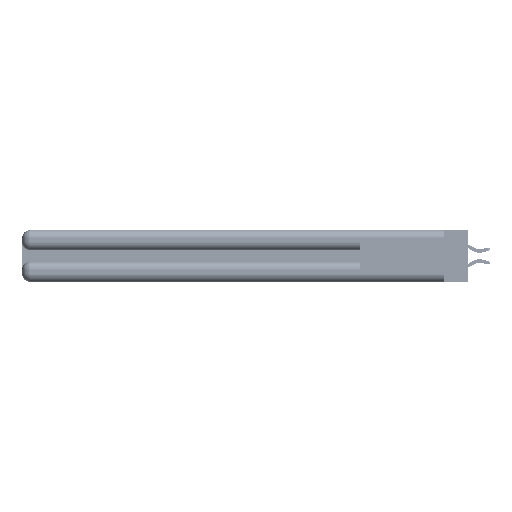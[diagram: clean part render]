
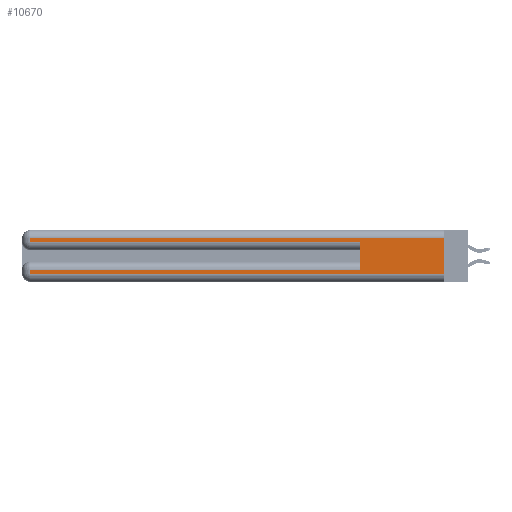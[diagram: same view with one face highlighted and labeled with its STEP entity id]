
A CAD part, left-side view. The second image highlights one B-rep face of the part: STEP entity #10670.
In plain terms, the highlighted planar face has unit normal (-1, 0, 0).
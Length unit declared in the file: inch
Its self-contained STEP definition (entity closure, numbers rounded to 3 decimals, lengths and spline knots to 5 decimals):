
#1679 = VECTOR ( 'NONE', #37091, 39.37008 ) ;
#2546 = VERTEX_POINT ( 'NONE', #47891 ) ;
#4419 = LINE ( 'NONE', #30171, #14768 ) ;
#5104 = ORIENTED_EDGE ( 'NONE', *, *, #55584, .T. ) ;
#5955 = LINE ( 'NONE', #19598, #27878 ) ;
#6009 = VERTEX_POINT ( 'NONE', #10461 ) ;
#6026 = LINE ( 'NONE', #41422, #39527 ) ;
#7440 = LINE ( 'NONE', #43760, #29347 ) ;
#9182 = EDGE_LOOP ( 'NONE', ( #13425, #17694, #44056, #31482, #10228, #5104, #28020, #56141 ) ) ;
#9237 = CARTESIAN_POINT ( 'NONE',  ( 0., 2.94, 0.06 ) ) ;
#10228 = ORIENTED_EDGE ( 'NONE', *, *, #19176, .F. ) ;
#10363 = VERTEX_POINT ( 'NONE', #9237 ) ;
#10461 = CARTESIAN_POINT ( 'NONE',  ( 0., 0.6, 0.285 ) ) ;
#10521 = VERTEX_POINT ( 'NONE', #23574 ) ;
#10670 = ADVANCED_FACE ( 'NONE', ( #22972 ), #11326, .F. ) ;
#11326 = PLANE ( 'NONE',  #25220 ) ;
#13425 = ORIENTED_EDGE ( 'NONE', *, *, #25751, .F. ) ;
#14768 = VECTOR ( 'NONE', #17001, 39.37008 ) ;
#15258 = VECTOR ( 'NONE', #37832, 39.37008 ) ;
#16600 = LINE ( 'NONE', #33447, #15258 ) ;
#16718 = VECTOR ( 'NONE', #22267, 39.37008 ) ;
#17001 = DIRECTION ( 'NONE',  ( 0., 1., 0. ) ) ;
#17694 = ORIENTED_EDGE ( 'NONE', *, *, #53744, .T. ) ;
#19176 = EDGE_CURVE ( 'NONE', #2546, #6009, #6026, .T. ) ;
#19598 = CARTESIAN_POINT ( 'NONE',  ( 0., 2.94, 0.37 ) ) ;
#20478 = VECTOR ( 'NONE', #41008, 39.37008 ) ;
#21703 = CARTESIAN_POINT ( 'NONE',  ( 0., 0., 0.31 ) ) ;
#22267 = DIRECTION ( 'NONE',  ( 0., -1., 0. ) ) ;
#22469 = CARTESIAN_POINT ( 'NONE',  ( 0., 0., 0.06 ) ) ;
#22972 = FACE_OUTER_BOUND ( 'NONE', #9182, .T. ) ;
#23574 = CARTESIAN_POINT ( 'NONE',  ( 0., 2.94, 0.31 ) ) ;
#23806 = VERTEX_POINT ( 'NONE', #30714 ) ;
#23983 = CARTESIAN_POINT ( 'NONE',  ( 0., 2.94, 0.085 ) ) ;
#23995 = DIRECTION ( 'NONE',  ( 0., 0., -1. ) ) ;
#24495 = CARTESIAN_POINT ( 'NONE',  ( 0., 0., 0.37 ) ) ;
#25220 = AXIS2_PLACEMENT_3D ( 'NONE', #24495, #55102, #28906 ) ;
#25751 = EDGE_CURVE ( 'NONE', #33388, #52364, #16600, .T. ) ;
#27878 = VECTOR ( 'NONE', #23995, 39.37008 ) ;
#28020 = ORIENTED_EDGE ( 'NONE', *, *, #45472, .T. ) ;
#28379 = LINE ( 'NONE', #52677, #16718 ) ;
#28906 = DIRECTION ( 'NONE',  ( 0., 0., -1. ) ) ;
#29347 = VECTOR ( 'NONE', #48147, 39.37008 ) ;
#30171 = CARTESIAN_POINT ( 'NONE',  ( 0., 0., 0.085 ) ) ;
#30199 = EDGE_CURVE ( 'NONE', #10363, #52364, #36605, .T. ) ;
#30714 = CARTESIAN_POINT ( 'NONE',  ( 0., 2.94, 0.285 ) ) ;
#31482 = ORIENTED_EDGE ( 'NONE', *, *, #39135, .T. ) ;
#32717 = CARTESIAN_POINT ( 'NONE',  ( 0., 0., 0.06 ) ) ;
#33388 = VERTEX_POINT ( 'NONE', #21703 ) ;
#33447 = CARTESIAN_POINT ( 'NONE',  ( 0., 0., 0.37 ) ) ;
#36557 = CARTESIAN_POINT ( 'NONE',  ( 0., 2.94, 0.37 ) ) ;
#36605 = LINE ( 'NONE', #32717, #1679 ) ;
#37091 = DIRECTION ( 'NONE',  ( 0., -1., 0. ) ) ;
#37559 = EDGE_CURVE ( 'NONE', #10521, #23806, #5955, .T. ) ;
#37832 = DIRECTION ( 'NONE',  ( 0., 0., -1. ) ) ;
#39135 = EDGE_CURVE ( 'NONE', #23806, #6009, #28379, .T. ) ;
#39527 = VECTOR ( 'NONE', #45838, 39.37008 ) ;
#41008 = DIRECTION ( 'NONE',  ( 0., 0., -1. ) ) ;
#41422 = CARTESIAN_POINT ( 'NONE',  ( 0., 0.6, 0.145 ) ) ;
#42746 = VERTEX_POINT ( 'NONE', #23983 ) ;
#43760 = CARTESIAN_POINT ( 'NONE',  ( 0., 0., 0.31 ) ) ;
#44056 = ORIENTED_EDGE ( 'NONE', *, *, #37559, .T. ) ;
#45472 = EDGE_CURVE ( 'NONE', #42746, #10363, #55371, .T. ) ;
#45838 = DIRECTION ( 'NONE',  ( 0., 0., 1. ) ) ;
#47891 = CARTESIAN_POINT ( 'NONE',  ( 0., 0.6, 0.085 ) ) ;
#48147 = DIRECTION ( 'NONE',  ( 0., 1., 0. ) ) ;
#52364 = VERTEX_POINT ( 'NONE', #22469 ) ;
#52677 = CARTESIAN_POINT ( 'NONE',  ( 0., 0., 0.285 ) ) ;
#53744 = EDGE_CURVE ( 'NONE', #33388, #10521, #7440, .T. ) ;
#55102 = DIRECTION ( 'NONE',  ( 1., 0., 0. ) ) ;
#55371 = LINE ( 'NONE', #36557, #20478 ) ;
#55584 = EDGE_CURVE ( 'NONE', #2546, #42746, #4419, .T. ) ;
#56141 = ORIENTED_EDGE ( 'NONE', *, *, #30199, .T. ) ;
